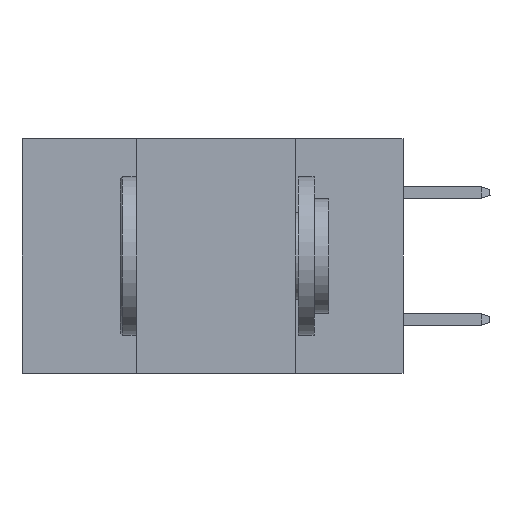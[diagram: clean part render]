
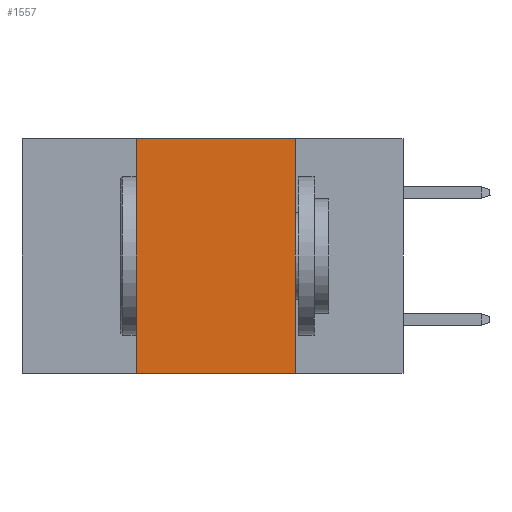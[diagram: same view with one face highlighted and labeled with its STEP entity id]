
A CAD part, left-side view. The second image highlights one B-rep face of the part: STEP entity #1557.
In plain terms, the highlighted planar face has unit normal (-1, 0, 0).
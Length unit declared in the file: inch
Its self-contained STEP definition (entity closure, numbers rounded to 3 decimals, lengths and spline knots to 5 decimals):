
#1557 = ADVANCED_FACE ( 'NONE', ( #19580 ), #38555, .F. ) ;
#5751 = AXIS2_PLACEMENT_3D ( 'NONE', #15791, #22523, #35408 ) ;
#6741 = DIRECTION ( 'NONE',  ( 0., -1., 0. ) ) ;
#8177 = VERTEX_POINT ( 'NONE', #17941 ) ;
#9150 = EDGE_CURVE ( 'NONE', #8177, #34240, #11561, .T. ) ;
#11561 = LINE ( 'NONE', #33889, #14809 ) ;
#11756 = LINE ( 'NONE', #24578, #17114 ) ;
#11955 = CARTESIAN_POINT ( 'NONE',  ( 0., 0.42, 0. ) ) ;
#12269 = ORIENTED_EDGE ( 'NONE', *, *, #16462, .F. ) ;
#14809 = VECTOR ( 'NONE', #27140, 39.37008 ) ;
#15791 = CARTESIAN_POINT ( 'NONE',  ( 0., 0.6, 0. ) ) ;
#16462 = EDGE_CURVE ( 'NONE', #23748, #21232, #32426, .T. ) ;
#16604 = VECTOR ( 'NONE', #6741, 39.37008 ) ;
#17114 = VECTOR ( 'NONE', #41280, 39.37008 ) ;
#17941 = CARTESIAN_POINT ( 'NONE',  ( 0., 0.42, -0.37 ) ) ;
#18992 = LINE ( 'NONE', #28691, #23251 ) ;
#19163 = CARTESIAN_POINT ( 'NONE',  ( 0., 0.6, 0. ) ) ;
#19580 = FACE_OUTER_BOUND ( 'NONE', #27193, .T. ) ;
#20989 = CARTESIAN_POINT ( 'NONE',  ( 0., 0.17, 0. ) ) ;
#21232 = VERTEX_POINT ( 'NONE', #20989 ) ;
#22523 = DIRECTION ( 'NONE',  ( 1., 0., 0. ) ) ;
#22825 = EDGE_CURVE ( 'NONE', #8177, #23748, #18992, .T. ) ;
#23251 = VECTOR ( 'NONE', #41569, 39.37008 ) ;
#23748 = VERTEX_POINT ( 'NONE', #11955 ) ;
#24578 = CARTESIAN_POINT ( 'NONE',  ( 0., 0.17, 0. ) ) ;
#27140 = DIRECTION ( 'NONE',  ( 0., -1., 0. ) ) ;
#27193 = EDGE_LOOP ( 'NONE', ( #34135, #12269, #33911, #39460 ) ) ;
#28691 = CARTESIAN_POINT ( 'NONE',  ( 0., 0.42, 0. ) ) ;
#32426 = LINE ( 'NONE', #19163, #16604 ) ;
#33665 = CARTESIAN_POINT ( 'NONE',  ( 0., 0.17, -0.37 ) ) ;
#33889 = CARTESIAN_POINT ( 'NONE',  ( 0., 0.6, -0.37 ) ) ;
#33911 = ORIENTED_EDGE ( 'NONE', *, *, #22825, .F. ) ;
#34135 = ORIENTED_EDGE ( 'NONE', *, *, #34376, .F. ) ;
#34240 = VERTEX_POINT ( 'NONE', #33665 ) ;
#34376 = EDGE_CURVE ( 'NONE', #21232, #34240, #11756, .T. ) ;
#35408 = DIRECTION ( 'NONE',  ( 0., 0., -1. ) ) ;
#38555 = PLANE ( 'NONE',  #5751 ) ;
#39460 = ORIENTED_EDGE ( 'NONE', *, *, #9150, .T. ) ;
#41280 = DIRECTION ( 'NONE',  ( 0., 0., -1. ) ) ;
#41569 = DIRECTION ( 'NONE',  ( 0., 0., 1. ) ) ;
